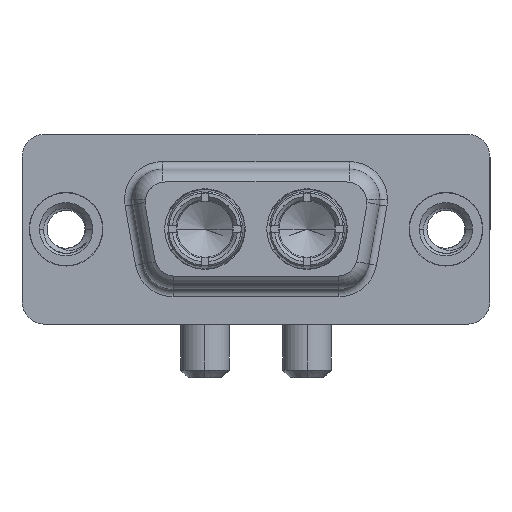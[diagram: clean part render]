
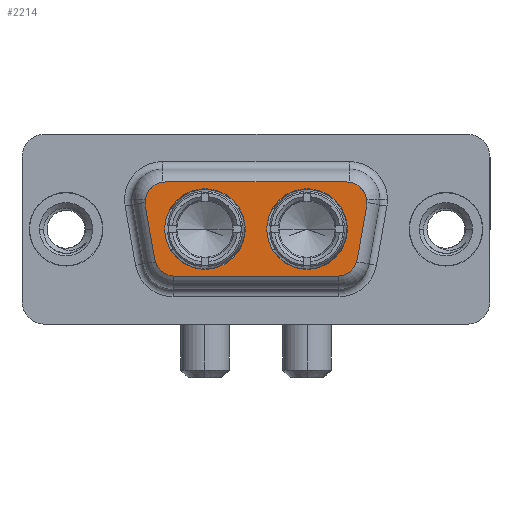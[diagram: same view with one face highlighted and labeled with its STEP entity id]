
A CAD part, top view. The second image highlights one B-rep face of the part: STEP entity #2214.
In plain terms, the highlighted planar face has unit normal (0, 0, 1).
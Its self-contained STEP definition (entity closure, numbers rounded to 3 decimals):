
#62 = CARTESIAN_POINT ( 'NONE',  ( 7.167, -3.1, 6.2 ) ) ;
#83 = DIRECTION ( 'NONE',  ( 0., 0., 1. ) ) ;
#396 = ORIENTED_EDGE ( 'NONE', *, *, #2501, .T. ) ;
#425 = CIRCLE ( 'NONE', #5125, 2.65 ) ;
#482 = EDGE_CURVE ( 'NONE', #4529, #4729, #7868, .T. ) ;
#537 = CARTESIAN_POINT ( 'NONE',  ( 5.221, 1.516, 6.2 ) ) ;
#560 = EDGE_CURVE ( 'NONE', #4574, #5988, #1592, .T. ) ;
#682 = EDGE_CURVE ( 'NONE', #7133, #8749, #3763, .T. ) ;
#773 = ORIENTED_EDGE ( 'NONE', *, *, #1306, .F. ) ;
#852 = ORIENTED_EDGE ( 'NONE', *, *, #3639, .T. ) ;
#860 = EDGE_LOOP ( 'NONE', ( #8451, #10679 ) ) ;
#913 = DIRECTION ( 'NONE',  ( 1., 0., 0. ) ) ;
#1164 = DIRECTION ( 'NONE',  ( 0.174, 0.985, 0. ) ) ;
#1196 = EDGE_CURVE ( 'NONE', #4071, #11980, #9058, .T. ) ;
#1306 = EDGE_CURVE ( 'NONE', #4729, #4529, #425, .T. ) ;
#1361 = ORIENTED_EDGE ( 'NONE', *, *, #2897, .T. ) ;
#1417 = CARTESIAN_POINT ( 'NONE',  ( 5.838, -1.984, 6.2 ) ) ;
#1509 = CARTESIAN_POINT ( 'NONE',  ( 17.833, -3.1, 6.2 ) ) ;
#1592 = CIRCLE ( 'NONE', #5519, 2.65 ) ;
#1751 = EDGE_CURVE ( 'NONE', #9674, #4071, #5829, .T. ) ;
#1759 = LINE ( 'NONE', #9020, #4805 ) ;
#1789 = DIRECTION ( 'NONE',  ( 0., 0., 1. ) ) ;
#1841 = DIRECTION ( 'NONE',  ( 1., 0., 0. ) ) ;
#1890 = CARTESIAN_POINT ( 'NONE',  ( 17.833, -1.75, 6.2 ) ) ;
#2214 = ADVANCED_FACE ( 'NONE', ( #6800, #7541, #7662 ), #5815, .F. ) ;
#2269 = ORIENTED_EDGE ( 'NONE', *, *, #5822, .T. ) ;
#2280 = ORIENTED_EDGE ( 'NONE', *, *, #2497, .T. ) ;
#2316 = ORIENTED_EDGE ( 'NONE', *, *, #1196, .T. ) ;
#2367 = CARTESIAN_POINT ( 'NONE',  ( 5.2, 1.75, 6.2 ) ) ;
#2454 = CARTESIAN_POINT ( 'NONE',  ( 19.162, -1.984, 6.2 ) ) ;
#2491 = DIRECTION ( 'NONE',  ( -1., 0., 0. ) ) ;
#2497 = EDGE_CURVE ( 'NONE', #11980, #10820, #1759, .T. ) ;
#2501 = EDGE_CURVE ( 'NONE', #8749, #4683, #6367, .T. ) ;
#2542 = ORIENTED_EDGE ( 'NONE', *, *, #682, .T. ) ;
#2656 = DIRECTION ( 'NONE',  ( -1., 0., 0. ) ) ;
#2838 = CIRCLE ( 'NONE', #10497, 2.65 ) ;
#2867 = DIRECTION ( 'NONE',  ( -1., 0., 0. ) ) ;
#2897 = EDGE_CURVE ( 'NONE', #10561, #3819, #6183, .T. ) ;
#2930 = DIRECTION ( 'NONE',  ( 0., 0., -1. ) ) ;
#2969 = CIRCLE ( 'NONE', #6517, 1.35 ) ;
#3040 = AXIS2_PLACEMENT_3D ( 'NONE', #6846, #8117, #11848 ) ;
#3430 = AXIS2_PLACEMENT_3D ( 'NONE', #1890, #8712, #10427 ) ;
#3550 = AXIS2_PLACEMENT_3D ( 'NONE', #6474, #8445, #2656 ) ;
#3639 = EDGE_CURVE ( 'NONE', #4683, #9674, #10305, .T. ) ;
#3729 = DIRECTION ( 'NONE',  ( 0., 0., 1. ) ) ;
#3763 = CIRCLE ( 'NONE', #11786, 1.35 ) ;
#3781 = VECTOR ( 'NONE', #10995, 1000. ) ;
#3819 = VERTEX_POINT ( 'NONE', #537 ) ;
#4026 = DIRECTION ( 'NONE',  ( -1., 0., 0. ) ) ;
#4071 = VERTEX_POINT ( 'NONE', #12131 ) ;
#4380 = CARTESIAN_POINT ( 'NONE',  ( 6.55, 3.1, 6.2 ) ) ;
#4529 = VERTEX_POINT ( 'NONE', #4687 ) ;
#4574 = VERTEX_POINT ( 'NONE', #8625 ) ;
#4683 = VERTEX_POINT ( 'NONE', #5913 ) ;
#4687 = CARTESIAN_POINT ( 'NONE',  ( 13.21, 0., 6.2 ) ) ;
#4729 = VERTEX_POINT ( 'NONE', #8002 ) ;
#4782 = CARTESIAN_POINT ( 'NONE',  ( 9.14, 0., 6.2 ) ) ;
#4805 = VECTOR ( 'NONE', #2491, 1000. ) ;
#5125 = AXIS2_PLACEMENT_3D ( 'NONE', #11480, #83, #10507 ) ;
#5284 = LINE ( 'NONE', #1417, #3781 ) ;
#5393 = ORIENTED_EDGE ( 'NONE', *, *, #482, .F. ) ;
#5447 = EDGE_CURVE ( 'NONE', #10820, #10561, #2969, .T. ) ;
#5519 = AXIS2_PLACEMENT_3D ( 'NONE', #10471, #3729, #913 ) ;
#5645 = CARTESIAN_POINT ( 'NONE',  ( 19.779, 1.516, 6.2 ) ) ;
#5815 = PLANE ( 'NONE',  #10286 ) ;
#5822 = EDGE_CURVE ( 'NONE', #3819, #7133, #5284, .T. ) ;
#5829 = LINE ( 'NONE', #5645, #6330 ) ;
#5913 = CARTESIAN_POINT ( 'NONE',  ( 17.833, -3.1, 6.2 ) ) ;
#5988 = VERTEX_POINT ( 'NONE', #7741 ) ;
#6183 = CIRCLE ( 'NONE', #3040, 1.35 ) ;
#6306 = EDGE_CURVE ( 'NONE', #5988, #4574, #2838, .T. ) ;
#6330 = VECTOR ( 'NONE', #1164, 1000. ) ;
#6367 = LINE ( 'NONE', #1509, #8744 ) ;
#6474 = CARTESIAN_POINT ( 'NONE',  ( 18.45, 1.75, 6.2 ) ) ;
#6517 = AXIS2_PLACEMENT_3D ( 'NONE', #6538, #11242, #7509 ) ;
#6538 = CARTESIAN_POINT ( 'NONE',  ( 6.55, 1.75, 6.2 ) ) ;
#6800 = FACE_BOUND ( 'NONE', #10062, .T. ) ;
#6806 = ORIENTED_EDGE ( 'NONE', *, *, #5447, .T. ) ;
#6846 = CARTESIAN_POINT ( 'NONE',  ( 6.55, 1.75, 6.2 ) ) ;
#6851 = DIRECTION ( 'NONE',  ( 0., 0., 1. ) ) ;
#6886 = AXIS2_PLACEMENT_3D ( 'NONE', #11212, #11390, #7475 ) ;
#7133 = VERTEX_POINT ( 'NONE', #8654 ) ;
#7475 = DIRECTION ( 'NONE',  ( 1., 0., 0. ) ) ;
#7509 = DIRECTION ( 'NONE',  ( 1., 0., 0. ) ) ;
#7541 = FACE_BOUND ( 'NONE', #860, .T. ) ;
#7662 = FACE_OUTER_BOUND ( 'NONE', #12015, .T. ) ;
#7741 = CARTESIAN_POINT ( 'NONE',  ( 6.49, 0., 6.2 ) ) ;
#7862 = ORIENTED_EDGE ( 'NONE', *, *, #1751, .T. ) ;
#7868 = CIRCLE ( 'NONE', #6886, 2.65 ) ;
#8002 = CARTESIAN_POINT ( 'NONE',  ( 18.51, 0., 6.2 ) ) ;
#8084 = CARTESIAN_POINT ( 'NONE',  ( 18.45, 3.1, 6.2 ) ) ;
#8117 = DIRECTION ( 'NONE',  ( 0., 0., 1. ) ) ;
#8445 = DIRECTION ( 'NONE',  ( 0., 0., 1. ) ) ;
#8451 = ORIENTED_EDGE ( 'NONE', *, *, #560, .F. ) ;
#8625 = CARTESIAN_POINT ( 'NONE',  ( 11.79, 0., 6.2 ) ) ;
#8654 = CARTESIAN_POINT ( 'NONE',  ( 5.838, -1.984, 6.2 ) ) ;
#8712 = DIRECTION ( 'NONE',  ( 0., 0., 1. ) ) ;
#8744 = VECTOR ( 'NONE', #10166, 1000. ) ;
#8749 = VERTEX_POINT ( 'NONE', #62 ) ;
#9020 = CARTESIAN_POINT ( 'NONE',  ( 6.55, 3.1, 6.2 ) ) ;
#9058 = CIRCLE ( 'NONE', #3550, 1.35 ) ;
#9674 = VERTEX_POINT ( 'NONE', #2454 ) ;
#10062 = EDGE_LOOP ( 'NONE', ( #773, #5393 ) ) ;
#10166 = DIRECTION ( 'NONE',  ( 1., 0., 0. ) ) ;
#10286 = AXIS2_PLACEMENT_3D ( 'NONE', #11278, #2930, #2867 ) ;
#10305 = CIRCLE ( 'NONE', #3430, 1.35 ) ;
#10427 = DIRECTION ( 'NONE',  ( -1., 0., 0. ) ) ;
#10471 = CARTESIAN_POINT ( 'NONE',  ( 9.14, 0., 6.2 ) ) ;
#10497 = AXIS2_PLACEMENT_3D ( 'NONE', #4782, #1789, #1841 ) ;
#10507 = DIRECTION ( 'NONE',  ( 1., 0., 0. ) ) ;
#10561 = VERTEX_POINT ( 'NONE', #2367 ) ;
#10657 = CARTESIAN_POINT ( 'NONE',  ( 7.167, -1.75, 6.2 ) ) ;
#10679 = ORIENTED_EDGE ( 'NONE', *, *, #6306, .F. ) ;
#10820 = VERTEX_POINT ( 'NONE', #4380 ) ;
#10995 = DIRECTION ( 'NONE',  ( 0.174, -0.985, 0. ) ) ;
#11212 = CARTESIAN_POINT ( 'NONE',  ( 15.86, 0., 6.2 ) ) ;
#11242 = DIRECTION ( 'NONE',  ( 0., 0., 1. ) ) ;
#11278 = CARTESIAN_POINT ( 'NONE',  ( 7.167, -1.75, 6.2 ) ) ;
#11390 = DIRECTION ( 'NONE',  ( 0., 0., 1. ) ) ;
#11480 = CARTESIAN_POINT ( 'NONE',  ( 15.86, 0., 6.2 ) ) ;
#11786 = AXIS2_PLACEMENT_3D ( 'NONE', #10657, #6851, #4026 ) ;
#11848 = DIRECTION ( 'NONE',  ( 1., 0., 0. ) ) ;
#11980 = VERTEX_POINT ( 'NONE', #8084 ) ;
#12015 = EDGE_LOOP ( 'NONE', ( #2542, #396, #852, #7862, #2316, #2280, #6806, #1361, #2269 ) ) ;
#12131 = CARTESIAN_POINT ( 'NONE',  ( 19.779, 1.516, 6.2 ) ) ;
